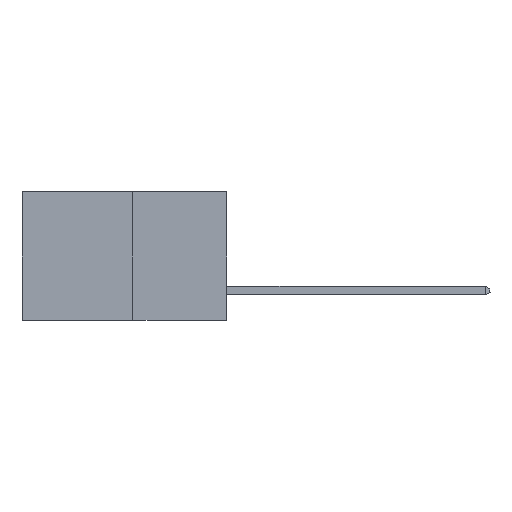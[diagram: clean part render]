
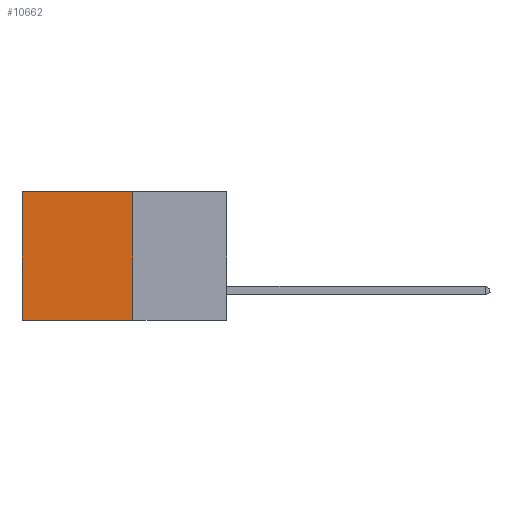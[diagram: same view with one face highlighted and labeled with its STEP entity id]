
A CAD part, left-side view. The second image highlights one B-rep face of the part: STEP entity #10662.
In plain terms, the highlighted planar face has unit normal (-1, 0, 0).
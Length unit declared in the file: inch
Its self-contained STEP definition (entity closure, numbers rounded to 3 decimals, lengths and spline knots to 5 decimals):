
#207 = VERTEX_POINT ( 'NONE', #9823 ) ;
#481 = CARTESIAN_POINT ( 'NONE',  ( 0.277, 0.59, -0.37 ) ) ;
#724 = DIRECTION ( 'NONE',  ( 0., 1., 0. ) ) ;
#917 = ORIENTED_EDGE ( 'NONE', *, *, #2348, .T. ) ;
#1199 = VERTEX_POINT ( 'NONE', #11245 ) ;
#1222 = DIRECTION ( 'NONE',  ( 1., 0., 0. ) ) ;
#1244 = ORIENTED_EDGE ( 'NONE', *, *, #10266, .T. ) ;
#1971 = AXIS2_PLACEMENT_3D ( 'NONE', #8210, #1222, #8256 ) ;
#2112 = FACE_OUTER_BOUND ( 'NONE', #3744, .T. ) ;
#2348 = EDGE_CURVE ( 'NONE', #3469, #207, #10087, .T. ) ;
#2725 = DIRECTION ( 'NONE',  ( 0., 1., 0. ) ) ;
#3080 = CARTESIAN_POINT ( 'NONE',  ( 0.277, 0.27, 0. ) ) ;
#3469 = VERTEX_POINT ( 'NONE', #9415 ) ;
#3621 = ORIENTED_EDGE ( 'NONE', *, *, #4230, .F. ) ;
#3744 = EDGE_LOOP ( 'NONE', ( #917, #6275, #3621, #1244 ) ) ;
#4179 = LINE ( 'NONE', #10724, #11722 ) ;
#4230 = EDGE_CURVE ( 'NONE', #4258, #1199, #8975, .T. ) ;
#4258 = VERTEX_POINT ( 'NONE', #3080 ) ;
#5977 = VECTOR ( 'NONE', #7843, 39.37008 ) ;
#6275 = ORIENTED_EDGE ( 'NONE', *, *, #12131, .F. ) ;
#7086 = VECTOR ( 'NONE', #7856, 39.37008 ) ;
#7089 = LINE ( 'NONE', #8798, #9171 ) ;
#7235 = PLANE ( 'NONE',  #1971 ) ;
#7843 = DIRECTION ( 'NONE',  ( 0., 0., -1. ) ) ;
#7856 = DIRECTION ( 'NONE',  ( 0., 0., -1. ) ) ;
#8210 = CARTESIAN_POINT ( 'NONE',  ( 0.277, 0.27, -0.37 ) ) ;
#8256 = DIRECTION ( 'NONE',  ( 0., 0., -1. ) ) ;
#8798 = CARTESIAN_POINT ( 'NONE',  ( 0.277, 0.27, -0.37 ) ) ;
#8975 = LINE ( 'NONE', #9573, #5977 ) ;
#9171 = VECTOR ( 'NONE', #724, 39.37008 ) ;
#9415 = CARTESIAN_POINT ( 'NONE',  ( 0.277, 0.59, 0. ) ) ;
#9573 = CARTESIAN_POINT ( 'NONE',  ( 0.277, 0.27, -0.37 ) ) ;
#9823 = CARTESIAN_POINT ( 'NONE',  ( 0.277, 0.59, -0.37 ) ) ;
#10087 = LINE ( 'NONE', #481, #7086 ) ;
#10266 = EDGE_CURVE ( 'NONE', #4258, #3469, #4179, .T. ) ;
#10662 = ADVANCED_FACE ( 'NONE', ( #2112 ), #7235, .F. ) ;
#10724 = CARTESIAN_POINT ( 'NONE',  ( 0.277, 0.27, 0. ) ) ;
#11245 = CARTESIAN_POINT ( 'NONE',  ( 0.277, 0.27, -0.37 ) ) ;
#11722 = VECTOR ( 'NONE', #2725, 39.37008 ) ;
#12131 = EDGE_CURVE ( 'NONE', #1199, #207, #7089, .T. ) ;
